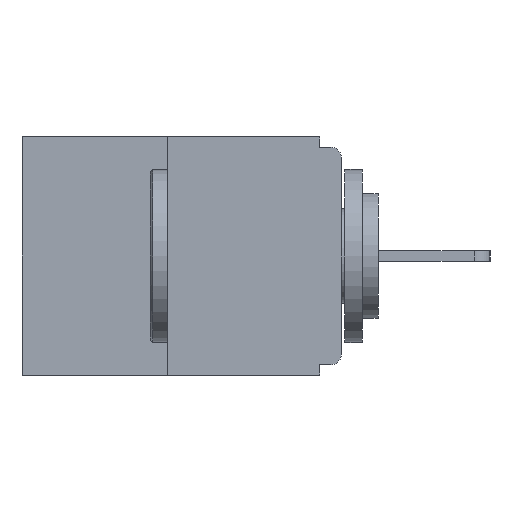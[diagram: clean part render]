
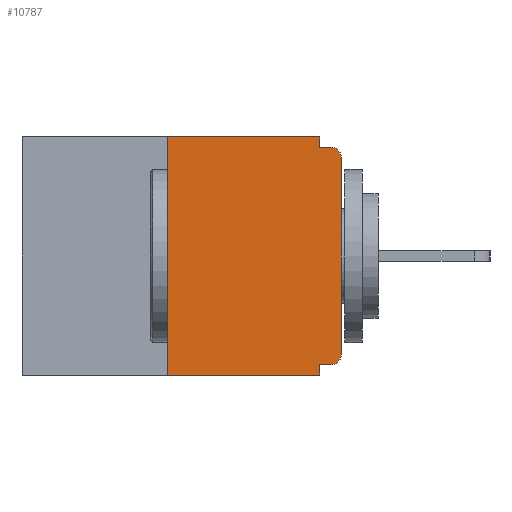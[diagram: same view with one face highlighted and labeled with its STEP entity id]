
A CAD part, left-side view. The second image highlights one B-rep face of the part: STEP entity #10787.
In plain terms, the highlighted planar face has unit normal (-1, 0, 0).
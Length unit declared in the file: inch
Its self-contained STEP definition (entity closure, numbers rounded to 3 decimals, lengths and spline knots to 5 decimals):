
#259 = CARTESIAN_POINT ( 'NONE',  ( 0., 0., -0.328 ) ) ;
#593 = CARTESIAN_POINT ( 'NONE',  ( 0., 0.015, -0.015 ) ) ;
#648 = CARTESIAN_POINT ( 'NONE',  ( 0., 0.015, -0.313 ) ) ;
#730 = FACE_OUTER_BOUND ( 'NONE', #7249, .T. ) ;
#733 = LINE ( 'NONE', #6658, #14814 ) ;
#1102 = VECTOR ( 'NONE', #14280, 39.37008 ) ;
#1440 = VERTEX_POINT ( 'NONE', #1572 ) ;
#1456 = AXIS2_PLACEMENT_3D ( 'NONE', #14448, #8847, #12330 ) ;
#1557 = ORIENTED_EDGE ( 'NONE', *, *, #6248, .T. ) ;
#1572 = CARTESIAN_POINT ( 'NONE',  ( 0., 0., -0.313 ) ) ;
#1762 = ORIENTED_EDGE ( 'NONE', *, *, #10360, .F. ) ;
#2089 = VERTEX_POINT ( 'NONE', #593 ) ;
#2271 = VERTEX_POINT ( 'NONE', #6625 ) ;
#2839 = ORIENTED_EDGE ( 'NONE', *, *, #13353, .T. ) ;
#2945 = VECTOR ( 'NONE', #10812, 39.37008 ) ;
#3726 = DIRECTION ( 'NONE',  ( 0., 0., -1. ) ) ;
#3756 = CARTESIAN_POINT ( 'NONE',  ( 0., 0.031, -0.015 ) ) ;
#4287 = CARTESIAN_POINT ( 'NONE',  ( 0., 0.031, -0.343 ) ) ;
#4295 = EDGE_CURVE ( 'NONE', #8181, #9582, #11381, .T. ) ;
#4308 = DIRECTION ( 'NONE',  ( 0., 0., 1. ) ) ;
#4408 = ORIENTED_EDGE ( 'NONE', *, *, #7876, .F. ) ;
#4598 = CARTESIAN_POINT ( 'NONE',  ( 0., 0., -0.015 ) ) ;
#4920 = DIRECTION ( 'NONE',  ( 0., 0., -1. ) ) ;
#5152 = DIRECTION ( 'NONE',  ( 0., 0., -1. ) ) ;
#5191 = VERTEX_POINT ( 'NONE', #3756 ) ;
#5263 = DIRECTION ( 'NONE',  ( 0., -1., 0. ) ) ;
#5489 = LINE ( 'NONE', #10480, #1102 ) ;
#5493 = VERTEX_POINT ( 'NONE', #14645 ) ;
#5610 = LINE ( 'NONE', #15685, #16020 ) ;
#5740 = AXIS2_PLACEMENT_3D ( 'NONE', #12191, #13476, #14714 ) ;
#5984 = CIRCLE ( 'NONE', #10938, 0.015 ) ;
#6014 = DIRECTION ( 'NONE',  ( -1., 0., 0. ) ) ;
#6248 = EDGE_CURVE ( 'NONE', #1440, #2271, #5489, .T. ) ;
#6501 = VECTOR ( 'NONE', #8210, 39.37008 ) ;
#6625 = CARTESIAN_POINT ( 'NONE',  ( 0., 0., -0.03 ) ) ;
#6658 = CARTESIAN_POINT ( 'NONE',  ( 0., 0.46, -0.343 ) ) ;
#6694 = VERTEX_POINT ( 'NONE', #15734 ) ;
#7249 = EDGE_LOOP ( 'NONE', ( #8764, #1762, #12348, #13851, #14358, #11130, #1557, #2839, #4408, #7982 ) ) ;
#7378 = CARTESIAN_POINT ( 'NONE',  ( 0., 0.031, 0. ) ) ;
#7716 = VERTEX_POINT ( 'NONE', #4287 ) ;
#7867 = CARTESIAN_POINT ( 'NONE',  ( 0., 0.25, 0. ) ) ;
#7876 = EDGE_CURVE ( 'NONE', #5191, #2089, #15658, .T. ) ;
#7982 = ORIENTED_EDGE ( 'NONE', *, *, #8005, .F. ) ;
#8005 = EDGE_CURVE ( 'NONE', #9582, #5191, #13634, .T. ) ;
#8181 = VERTEX_POINT ( 'NONE', #7867 ) ;
#8210 = DIRECTION ( 'NONE',  ( 0., 1., 0. ) ) ;
#8635 = CARTESIAN_POINT ( 'NONE',  ( 0., 0.46, 0. ) ) ;
#8764 = ORIENTED_EDGE ( 'NONE', *, *, #4295, .F. ) ;
#8769 = LINE ( 'NONE', #15400, #10345 ) ;
#8847 = DIRECTION ( 'NONE',  ( 1., 0., 0. ) ) ;
#9505 = VECTOR ( 'NONE', #4920, 39.37008 ) ;
#9582 = VERTEX_POINT ( 'NONE', #13202 ) ;
#10345 = VECTOR ( 'NONE', #5152, 39.37008 ) ;
#10360 = EDGE_CURVE ( 'NONE', #6694, #8181, #5610, .T. ) ;
#10480 = CARTESIAN_POINT ( 'NONE',  ( 0., 0., 0. ) ) ;
#10486 = DIRECTION ( 'NONE',  ( 0., -1., 0. ) ) ;
#10713 = PLANE ( 'NONE',  #1456 ) ;
#10787 = ADVANCED_FACE ( 'NONE', ( #730 ), #10713, .F. ) ;
#10812 = DIRECTION ( 'NONE',  ( 0., -1., 0. ) ) ;
#10932 = EDGE_CURVE ( 'NONE', #11909, #7716, #8769, .T. ) ;
#10938 = AXIS2_PLACEMENT_3D ( 'NONE', #648, #6014, #3726 ) ;
#11130 = ORIENTED_EDGE ( 'NONE', *, *, #14102, .T. ) ;
#11381 = LINE ( 'NONE', #8635, #14625 ) ;
#11909 = VERTEX_POINT ( 'NONE', #12746 ) ;
#12191 = CARTESIAN_POINT ( 'NONE',  ( 0., 0.015, -0.03 ) ) ;
#12330 = DIRECTION ( 'NONE',  ( 0., 0., -1. ) ) ;
#12348 = ORIENTED_EDGE ( 'NONE', *, *, #13591, .T. ) ;
#12746 = CARTESIAN_POINT ( 'NONE',  ( 0., 0.031, -0.328 ) ) ;
#13202 = CARTESIAN_POINT ( 'NONE',  ( 0., 0.031, 0. ) ) ;
#13353 = EDGE_CURVE ( 'NONE', #2271, #2089, #14327, .T. ) ;
#13476 = DIRECTION ( 'NONE',  ( -1., 0., 0. ) ) ;
#13579 = EDGE_CURVE ( 'NONE', #5493, #11909, #14044, .T. ) ;
#13591 = EDGE_CURVE ( 'NONE', #6694, #7716, #733, .T. ) ;
#13634 = LINE ( 'NONE', #7378, #9505 ) ;
#13851 = ORIENTED_EDGE ( 'NONE', *, *, #10932, .F. ) ;
#14044 = LINE ( 'NONE', #259, #6501 ) ;
#14102 = EDGE_CURVE ( 'NONE', #5493, #1440, #5984, .T. ) ;
#14280 = DIRECTION ( 'NONE',  ( 0., 0., 1. ) ) ;
#14327 = CIRCLE ( 'NONE', #5740, 0.015 ) ;
#14358 = ORIENTED_EDGE ( 'NONE', *, *, #13579, .F. ) ;
#14448 = CARTESIAN_POINT ( 'NONE',  ( 0., 0.46, 0. ) ) ;
#14625 = VECTOR ( 'NONE', #5263, 39.37008 ) ;
#14645 = CARTESIAN_POINT ( 'NONE',  ( 0., 0.015, -0.328 ) ) ;
#14714 = DIRECTION ( 'NONE',  ( 0., 0., -1. ) ) ;
#14814 = VECTOR ( 'NONE', #10486, 39.37008 ) ;
#15400 = CARTESIAN_POINT ( 'NONE',  ( 0., 0.031, -0.343 ) ) ;
#15658 = LINE ( 'NONE', #4598, #2945 ) ;
#15685 = CARTESIAN_POINT ( 'NONE',  ( 0., 0.25, 0. ) ) ;
#15734 = CARTESIAN_POINT ( 'NONE',  ( 0., 0.25, -0.343 ) ) ;
#16020 = VECTOR ( 'NONE', #4308, 39.37008 ) ;
